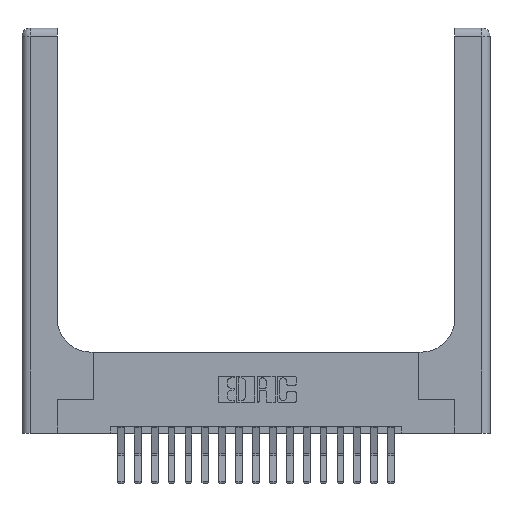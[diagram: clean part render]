
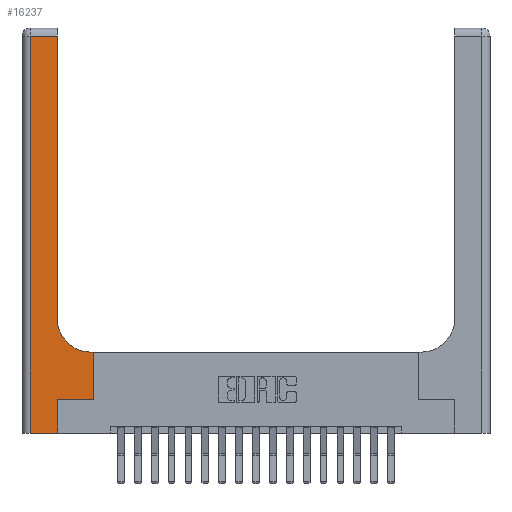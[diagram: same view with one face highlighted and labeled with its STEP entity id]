
A CAD part, top view. The second image highlights one B-rep face of the part: STEP entity #16237.
In plain terms, the highlighted planar face has unit normal (0, 0, 1).
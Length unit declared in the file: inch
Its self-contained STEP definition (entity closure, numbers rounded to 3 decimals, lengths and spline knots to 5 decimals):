
#275 = AXIS2_PLACEMENT_3D ( 'NONE', #921, #17558, #2039 ) ;
#341 = ORIENTED_EDGE ( 'NONE', *, *, #16811, .T. ) ;
#377 = DIRECTION ( 'NONE',  ( 1., 0., 0. ) ) ;
#921 = CARTESIAN_POINT ( 'NONE',  ( 0.51, 0.85, 0.37 ) ) ;
#966 = LINE ( 'NONE', #13426, #6083 ) ;
#981 = CARTESIAN_POINT ( 'NONE',  ( 0.265, 0., 0.37 ) ) ;
#1708 = DIRECTION ( 'NONE',  ( -1., 0., 0. ) ) ;
#2024 = DIRECTION ( 'NONE',  ( 0., 0., -1. ) ) ;
#2039 = DIRECTION ( 'NONE',  ( 1., 0., 0. ) ) ;
#2107 = ORIENTED_EDGE ( 'NONE', *, *, #13876, .T. ) ;
#2358 = EDGE_CURVE ( 'NONE', #10121, #7352, #6463, .T. ) ;
#2448 = CARTESIAN_POINT ( 'NONE',  ( 0.06, 3., 0.37 ) ) ;
#2509 = EDGE_CURVE ( 'NONE', #7352, #8370, #18469, .T. ) ;
#2957 = DIRECTION ( 'NONE',  ( 0., 1., 0. ) ) ;
#3532 = CARTESIAN_POINT ( 'NONE',  ( 0., 0., 0.37 ) ) ;
#3636 = VERTEX_POINT ( 'NONE', #17727 ) ;
#3932 = ORIENTED_EDGE ( 'NONE', *, *, #7326, .T. ) ;
#4023 = DIRECTION ( 'NONE',  ( 0., 1., 0. ) ) ;
#4156 = VECTOR ( 'NONE', #12691, 39.37008 ) ;
#4220 = EDGE_CURVE ( 'NONE', #15449, #3636, #966, .T. ) ;
#4327 = ORIENTED_EDGE ( 'NONE', *, *, #2358, .T. ) ;
#4338 = VECTOR ( 'NONE', #6392, 39.37008 ) ;
#4760 = CARTESIAN_POINT ( 'NONE',  ( 0.26, 2.94, 0.37 ) ) ;
#6083 = VECTOR ( 'NONE', #4023, 39.37008 ) ;
#6244 = EDGE_CURVE ( 'NONE', #15345, #16145, #9048, .T. ) ;
#6392 = DIRECTION ( 'NONE',  ( 1., 0., 0. ) ) ;
#6416 = VECTOR ( 'NONE', #1708, 39.37008 ) ;
#6448 = CARTESIAN_POINT ( 'NONE',  ( 0.265, 0., 0.37 ) ) ;
#6463 = CIRCLE ( 'NONE', #275, 0.25 ) ;
#6827 = ORIENTED_EDGE ( 'NONE', *, *, #17392, .T. ) ;
#7085 = CARTESIAN_POINT ( 'NONE',  ( 0.265, 0.25, 0.37 ) ) ;
#7209 = ORIENTED_EDGE ( 'NONE', *, *, #17410, .T. ) ;
#7326 = EDGE_CURVE ( 'NONE', #3636, #10121, #18165, .T. ) ;
#7352 = VERTEX_POINT ( 'NONE', #17964 ) ;
#7442 = DIRECTION ( 'NONE',  ( -1., 0., 0. ) ) ;
#8351 = FACE_OUTER_BOUND ( 'NONE', #14916, .T. ) ;
#8370 = VERTEX_POINT ( 'NONE', #4760 ) ;
#9048 = LINE ( 'NONE', #2448, #10725 ) ;
#9362 = CARTESIAN_POINT ( 'NONE',  ( 0., 2.94, 0.37 ) ) ;
#9745 = CARTESIAN_POINT ( 'NONE',  ( 0.06, 2.94, 0.37 ) ) ;
#9787 = CARTESIAN_POINT ( 'NONE',  ( 0., 3., 0.37 ) ) ;
#9973 = PLANE ( 'NONE',  #14483 ) ;
#10121 = VERTEX_POINT ( 'NONE', #19436 ) ;
#10184 = VERTEX_POINT ( 'NONE', #7085 ) ;
#10236 = ORIENTED_EDGE ( 'NONE', *, *, #2509, .T. ) ;
#10714 = CARTESIAN_POINT ( 'NONE',  ( 0.26, 3., 0.37 ) ) ;
#10725 = VECTOR ( 'NONE', #11552, 39.37008 ) ;
#11083 = VECTOR ( 'NONE', #7442, 39.37008 ) ;
#11212 = LINE ( 'NONE', #12646, #11305 ) ;
#11300 = LINE ( 'NONE', #3532, #4338 ) ;
#11305 = VECTOR ( 'NONE', #377, 39.37008 ) ;
#11552 = DIRECTION ( 'NONE',  ( 0., -1., 0. ) ) ;
#11745 = CARTESIAN_POINT ( 'NONE',  ( 0.26, 0.6, 0.37 ) ) ;
#12646 = CARTESIAN_POINT ( 'NONE',  ( 0.265, 0.25, 0.37 ) ) ;
#12691 = DIRECTION ( 'NONE',  ( 0., 1., 0. ) ) ;
#13426 = CARTESIAN_POINT ( 'NONE',  ( 0.528, 0.25, 0.37 ) ) ;
#13876 = EDGE_CURVE ( 'NONE', #16145, #17829, #11300, .T. ) ;
#13911 = ORIENTED_EDGE ( 'NONE', *, *, #6244, .T. ) ;
#14483 = AXIS2_PLACEMENT_3D ( 'NONE', #9787, #2024, #14589 ) ;
#14589 = DIRECTION ( 'NONE',  ( -1., 0., 0. ) ) ;
#14916 = EDGE_LOOP ( 'NONE', ( #10236, #6827, #13911, #2107, #341, #7209, #18092, #3932, #4327 ) ) ;
#15345 = VERTEX_POINT ( 'NONE', #9745 ) ;
#15449 = VERTEX_POINT ( 'NONE', #20134 ) ;
#15708 = LINE ( 'NONE', #9362, #6416 ) ;
#16025 = CARTESIAN_POINT ( 'NONE',  ( 0.06, 0., 0.37 ) ) ;
#16145 = VERTEX_POINT ( 'NONE', #16025 ) ;
#16237 = ADVANCED_FACE ( 'NONE', ( #8351 ), #9973, .F. ) ;
#16811 = EDGE_CURVE ( 'NONE', #17829, #10184, #17270, .T. ) ;
#17270 = LINE ( 'NONE', #6448, #4156 ) ;
#17392 = EDGE_CURVE ( 'NONE', #8370, #15345, #15708, .T. ) ;
#17410 = EDGE_CURVE ( 'NONE', #10184, #15449, #11212, .T. ) ;
#17558 = DIRECTION ( 'NONE',  ( 0., 0., -1. ) ) ;
#17727 = CARTESIAN_POINT ( 'NONE',  ( 0.528, 0.6, 0.37 ) ) ;
#17829 = VERTEX_POINT ( 'NONE', #981 ) ;
#17964 = CARTESIAN_POINT ( 'NONE',  ( 0.26, 0.85, 0.37 ) ) ;
#18092 = ORIENTED_EDGE ( 'NONE', *, *, #4220, .T. ) ;
#18165 = LINE ( 'NONE', #11745, #11083 ) ;
#18469 = LINE ( 'NONE', #10714, #18908 ) ;
#18908 = VECTOR ( 'NONE', #2957, 39.37008 ) ;
#19436 = CARTESIAN_POINT ( 'NONE',  ( 0.51, 0.6, 0.37 ) ) ;
#20134 = CARTESIAN_POINT ( 'NONE',  ( 0.528, 0.25, 0.37 ) ) ;
